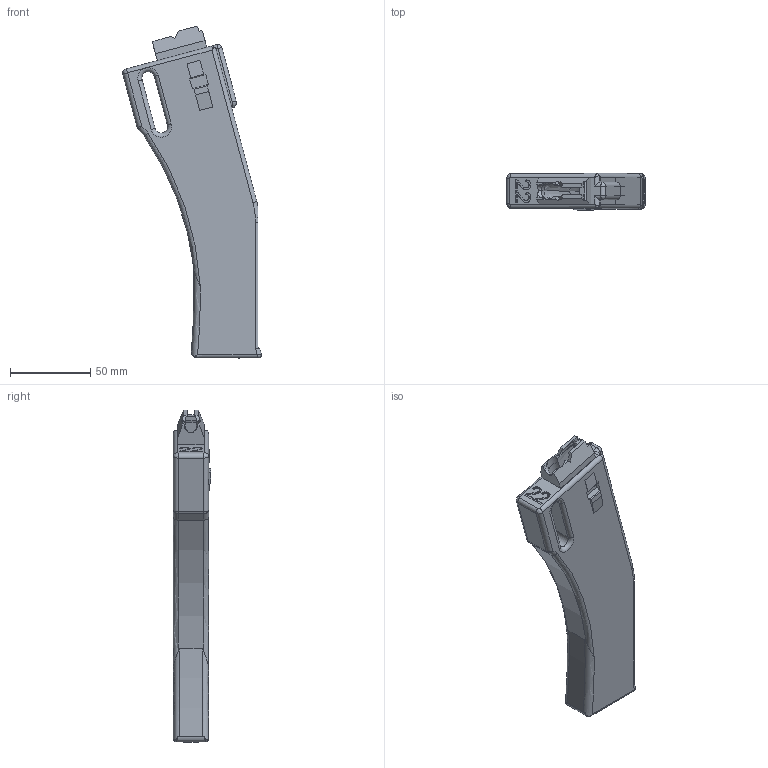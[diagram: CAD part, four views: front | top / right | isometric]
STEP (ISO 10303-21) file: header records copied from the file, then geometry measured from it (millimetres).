
FILE_DESCRIPTION(/* description */ (''),/* implementation_level */ '2;1');
FILE_NAME(/* name */ 'ar1522mag.step',/* time_stamp */ '2021-10-16T18:39:57-04:00',/* author */ (''),/* organization */ (''),/* preprocessor_version */ 'ST-DEVELOPER v18.1',/* originating_system */ 'Autodesk Translation Framework v10.10.0.1391',/* authorisation */ '');
FILE_SCHEMA (('AUTOMOTIVE_DESIGN { 1 0 10303 214 3 1 1 }'));
Length unit declared in the file: millimetre
Products named in the file (2): mag untested; BodyCombined-new
Assembly tree (1 placements, depth 2):
  mag untested
    BodyCombined-new
Bounding box: 86.55 x 23.32 x 207.37 mm (x, y, z)
Volume: 157929.3 mm3; surface area: 45731.8 mm2
Topology: 1 solids, 3 shells, 342 faces, 908 edges, 573 vertices
Faces by surface type: plane 126, bspline 124, cylinder 66, torus 12, cone 10, sphere 4
Entity records: 14311 total; most frequent: CARTESIAN_POINT 6604, ORIENTED_EDGE 1808, DIRECTION 1261, EDGE_CURVE 904, VERTEX_POINT 573, AXIS2_PLACEMENT_3D 436, LINE 389, VECTOR 389
